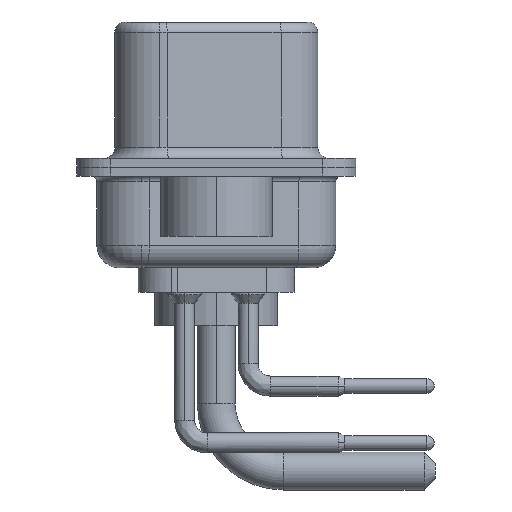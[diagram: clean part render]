
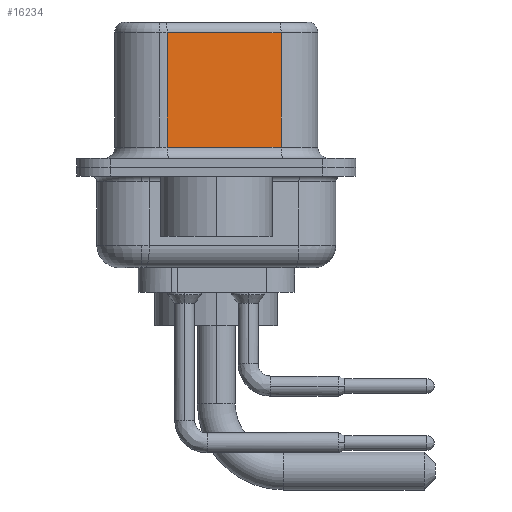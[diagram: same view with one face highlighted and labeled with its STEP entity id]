
A CAD part, left-side view. The second image highlights one B-rep face of the part: STEP entity #16234.
In plain terms, the highlighted planar face has unit normal (-0.985, -0.174, 0).
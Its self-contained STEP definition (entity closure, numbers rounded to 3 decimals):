
#238 = VERTEX_POINT ( 'NONE', #4867 ) ;
#533 = LINE ( 'NONE', #3824, #10241 ) ;
#1018 = AXIS2_PLACEMENT_3D ( 'NONE', #20238, #21722, #4716 ) ;
#3713 = VECTOR ( 'NONE', #5665, 1000. ) ;
#3824 = CARTESIAN_POINT ( 'NONE',  ( 4.555, -2.897, 0.9 ) ) ;
#4716 = DIRECTION ( 'NONE',  ( -0.174, 0.985, 0. ) ) ;
#4867 = CARTESIAN_POINT ( 'NONE',  ( 3.655, 2.203, 6.02 ) ) ;
#5038 = CARTESIAN_POINT ( 'NONE',  ( 3.655, 2.203, 0.9 ) ) ;
#5247 = CARTESIAN_POINT ( 'NONE',  ( 3.655, 2.203, 6.52 ) ) ;
#5665 = DIRECTION ( 'NONE',  ( 0., 0., -1. ) ) ;
#6417 = PLANE ( 'NONE',  #1018 ) ;
#7051 = LINE ( 'NONE', #5247, #14725 ) ;
#8233 = FACE_OUTER_BOUND ( 'NONE', #17731, .T. ) ;
#8844 = EDGE_CURVE ( 'NONE', #17922, #10326, #14280, .T. ) ;
#9322 = EDGE_CURVE ( 'NONE', #22330, #10326, #533, .T. ) ;
#10241 = VECTOR ( 'NONE', #14364, 1000. ) ;
#10326 = VERTEX_POINT ( 'NONE', #16863 ) ;
#10921 = ORIENTED_EDGE ( 'NONE', *, *, #9322, .T. ) ;
#10995 = CARTESIAN_POINT ( 'NONE',  ( 4.555, -2.897, 6.02 ) ) ;
#12020 = ORIENTED_EDGE ( 'NONE', *, *, #18740, .T. ) ;
#12476 = DIRECTION ( 'NONE',  ( -0.174, 0.985, 0. ) ) ;
#13087 = CARTESIAN_POINT ( 'NONE',  ( 4.555, -2.897, 6.02 ) ) ;
#14280 = LINE ( 'NONE', #21182, #3713 ) ;
#14364 = DIRECTION ( 'NONE',  ( 0.174, -0.985, 0. ) ) ;
#14725 = VECTOR ( 'NONE', #20863, 1000. ) ;
#15015 = EDGE_CURVE ( 'NONE', #238, #22330, #7051, .T. ) ;
#16234 = ADVANCED_FACE ( 'NONE', ( #8233 ), #6417, .F. ) ;
#16863 = CARTESIAN_POINT ( 'NONE',  ( 4.555, -2.897, 0.9 ) ) ;
#17731 = EDGE_LOOP ( 'NONE', ( #20442, #12020, #21752, #10921 ) ) ;
#17922 = VERTEX_POINT ( 'NONE', #13087 ) ;
#18740 = EDGE_CURVE ( 'NONE', #17922, #238, #19146, .T. ) ;
#19146 = LINE ( 'NONE', #10995, #20640 ) ;
#20238 = CARTESIAN_POINT ( 'NONE',  ( 4.555, -2.897, 6.52 ) ) ;
#20442 = ORIENTED_EDGE ( 'NONE', *, *, #8844, .F. ) ;
#20640 = VECTOR ( 'NONE', #12476, 1000. ) ;
#20863 = DIRECTION ( 'NONE',  ( 0., 0., -1. ) ) ;
#21182 = CARTESIAN_POINT ( 'NONE',  ( 4.555, -2.897, 6.52 ) ) ;
#21722 = DIRECTION ( 'NONE',  ( 0.985, 0.174, 0. ) ) ;
#21752 = ORIENTED_EDGE ( 'NONE', *, *, #15015, .T. ) ;
#22330 = VERTEX_POINT ( 'NONE', #5038 ) ;
